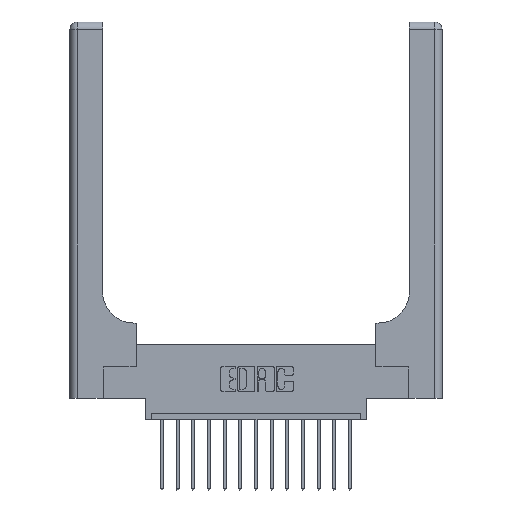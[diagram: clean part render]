
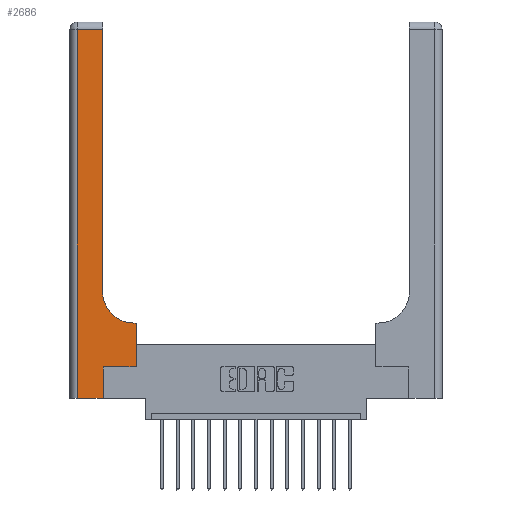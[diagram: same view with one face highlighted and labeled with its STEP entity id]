
A CAD part, top view. The second image highlights one B-rep face of the part: STEP entity #2686.
In plain terms, the highlighted planar face has unit normal (0, 0, 1).
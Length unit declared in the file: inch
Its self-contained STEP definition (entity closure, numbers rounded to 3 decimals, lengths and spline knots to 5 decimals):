
#4 = CARTESIAN_POINT ( 'NONE',  ( 0.26, 0.85, 0.37 ) ) ;
#49 = CARTESIAN_POINT ( 'NONE',  ( 0.06, 2.94, 0.37 ) ) ;
#787 = VERTEX_POINT ( 'NONE', #13604 ) ;
#789 = VERTEX_POINT ( 'NONE', #10816 ) ;
#888 = ORIENTED_EDGE ( 'NONE', *, *, #16746, .T. ) ;
#2177 = CARTESIAN_POINT ( 'NONE',  ( 0.26, 0.6, 0.37 ) ) ;
#2686 = ADVANCED_FACE ( 'NONE', ( #10068 ), #7264, .F. ) ;
#2805 = VECTOR ( 'NONE', #7332, 39.37008 ) ;
#3044 = CARTESIAN_POINT ( 'NONE',  ( 0.06, 0., 0.37 ) ) ;
#3117 = ORIENTED_EDGE ( 'NONE', *, *, #6387, .T. ) ;
#3392 = CARTESIAN_POINT ( 'NONE',  ( 0.51, 0.85, 0.37 ) ) ;
#3531 = EDGE_CURVE ( 'NONE', #9995, #789, #8189, .T. ) ;
#3611 = LINE ( 'NONE', #2177, #8663 ) ;
#4283 = VECTOR ( 'NONE', #16261, 39.37008 ) ;
#4434 = ORIENTED_EDGE ( 'NONE', *, *, #11020, .T. ) ;
#4485 = DIRECTION ( 'NONE',  ( 0., 0., -1. ) ) ;
#4554 = LINE ( 'NONE', #10054, #14372 ) ;
#4952 = ORIENTED_EDGE ( 'NONE', *, *, #7063, .T. ) ;
#5043 = DIRECTION ( 'NONE',  ( -1., 0., 0. ) ) ;
#5077 = VECTOR ( 'NONE', #5928, 39.37008 ) ;
#5084 = LINE ( 'NONE', #7872, #15592 ) ;
#5493 = CARTESIAN_POINT ( 'NONE',  ( 0., 0., 0.37 ) ) ;
#5574 = VERTEX_POINT ( 'NONE', #12785 ) ;
#5928 = DIRECTION ( 'NONE',  ( 0., 1., 0. ) ) ;
#6259 = VERTEX_POINT ( 'NONE', #3044 ) ;
#6260 = EDGE_CURVE ( 'NONE', #16279, #5574, #4554, .T. ) ;
#6387 = EDGE_CURVE ( 'NONE', #787, #11793, #17238, .T. ) ;
#6458 = DIRECTION ( 'NONE',  ( 1., 0., 0. ) ) ;
#6842 = DIRECTION ( 'NONE',  ( 1., 0., 0. ) ) ;
#7010 = LINE ( 'NONE', #9898, #5077 ) ;
#7063 = EDGE_CURVE ( 'NONE', #5574, #787, #3611, .T. ) ;
#7264 = PLANE ( 'NONE',  #14600 ) ;
#7332 = DIRECTION ( 'NONE',  ( 0., -1., 0. ) ) ;
#7616 = DIRECTION ( 'NONE',  ( 0., 0., -1. ) ) ;
#7872 = CARTESIAN_POINT ( 'NONE',  ( 0., 2.94, 0.37 ) ) ;
#8189 = LINE ( 'NONE', #12247, #4283 ) ;
#8609 = CARTESIAN_POINT ( 'NONE',  ( 0.06, 3., 0.37 ) ) ;
#8663 = VECTOR ( 'NONE', #5043, 39.37008 ) ;
#9502 = EDGE_LOOP ( 'NONE', ( #12442, #12484, #9921, #888, #12609, #4434, #13279, #4952, #3117 ) ) ;
#9518 = AXIS2_PLACEMENT_3D ( 'NONE', #3392, #7616, #6458 ) ;
#9626 = EDGE_CURVE ( 'NONE', #14619, #9735, #5084, .T. ) ;
#9735 = VERTEX_POINT ( 'NONE', #49 ) ;
#9898 = CARTESIAN_POINT ( 'NONE',  ( 0.26, 3., 0.37 ) ) ;
#9921 = ORIENTED_EDGE ( 'NONE', *, *, #12964, .T. ) ;
#9982 = DIRECTION ( 'NONE',  ( -1., 0., 0. ) ) ;
#9995 = VERTEX_POINT ( 'NONE', #10279 ) ;
#10054 = CARTESIAN_POINT ( 'NONE',  ( 0.528, 0.25, 0.37 ) ) ;
#10068 = FACE_OUTER_BOUND ( 'NONE', #9502, .T. ) ;
#10212 = CARTESIAN_POINT ( 'NONE',  ( 0.26, 2.94, 0.37 ) ) ;
#10279 = CARTESIAN_POINT ( 'NONE',  ( 0.265, 0., 0.37 ) ) ;
#10357 = VECTOR ( 'NONE', #13446, 39.37008 ) ;
#10816 = CARTESIAN_POINT ( 'NONE',  ( 0.265, 0.25, 0.37 ) ) ;
#11020 = EDGE_CURVE ( 'NONE', #789, #16279, #11096, .T. ) ;
#11096 = LINE ( 'NONE', #12371, #10357 ) ;
#11594 = LINE ( 'NONE', #5493, #13538 ) ;
#11606 = CARTESIAN_POINT ( 'NONE',  ( 0., 3., 0.37 ) ) ;
#11793 = VERTEX_POINT ( 'NONE', #4 ) ;
#12031 = EDGE_CURVE ( 'NONE', #11793, #14619, #7010, .T. ) ;
#12247 = CARTESIAN_POINT ( 'NONE',  ( 0.265, 0., 0.37 ) ) ;
#12371 = CARTESIAN_POINT ( 'NONE',  ( 0.265, 0.25, 0.37 ) ) ;
#12442 = ORIENTED_EDGE ( 'NONE', *, *, #12031, .T. ) ;
#12484 = ORIENTED_EDGE ( 'NONE', *, *, #9626, .T. ) ;
#12609 = ORIENTED_EDGE ( 'NONE', *, *, #3531, .T. ) ;
#12785 = CARTESIAN_POINT ( 'NONE',  ( 0.528, 0.6, 0.37 ) ) ;
#12964 = EDGE_CURVE ( 'NONE', #9735, #6259, #16684, .T. ) ;
#13279 = ORIENTED_EDGE ( 'NONE', *, *, #6260, .T. ) ;
#13446 = DIRECTION ( 'NONE',  ( 1., 0., 0. ) ) ;
#13538 = VECTOR ( 'NONE', #6842, 39.37008 ) ;
#13604 = CARTESIAN_POINT ( 'NONE',  ( 0.51, 0.6, 0.37 ) ) ;
#14056 = CARTESIAN_POINT ( 'NONE',  ( 0.528, 0.25, 0.37 ) ) ;
#14372 = VECTOR ( 'NONE', #15529, 39.37008 ) ;
#14600 = AXIS2_PLACEMENT_3D ( 'NONE', #11606, #4485, #9982 ) ;
#14619 = VERTEX_POINT ( 'NONE', #10212 ) ;
#14700 = DIRECTION ( 'NONE',  ( -1., 0., 0. ) ) ;
#15529 = DIRECTION ( 'NONE',  ( 0., 1., 0. ) ) ;
#15592 = VECTOR ( 'NONE', #14700, 39.37008 ) ;
#16261 = DIRECTION ( 'NONE',  ( 0., 1., 0. ) ) ;
#16279 = VERTEX_POINT ( 'NONE', #14056 ) ;
#16684 = LINE ( 'NONE', #8609, #2805 ) ;
#16746 = EDGE_CURVE ( 'NONE', #6259, #9995, #11594, .T. ) ;
#17238 = CIRCLE ( 'NONE', #9518, 0.25 ) ;
